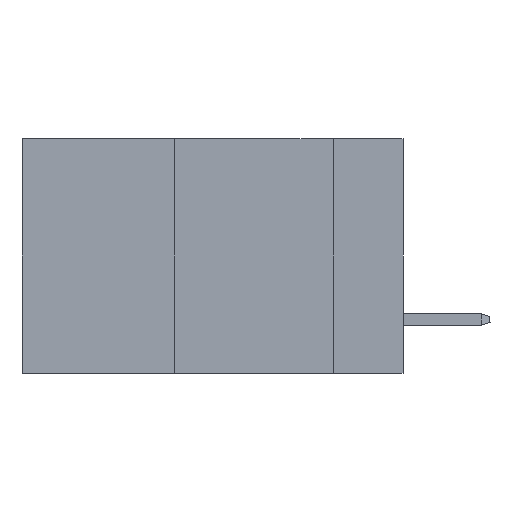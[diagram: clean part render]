
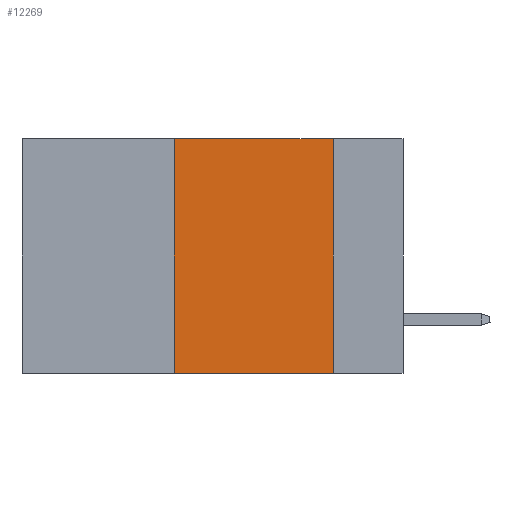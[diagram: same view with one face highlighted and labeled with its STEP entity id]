
A CAD part, left-side view. The second image highlights one B-rep face of the part: STEP entity #12269.
In plain terms, the highlighted planar face has unit normal (-1, 0, 0).
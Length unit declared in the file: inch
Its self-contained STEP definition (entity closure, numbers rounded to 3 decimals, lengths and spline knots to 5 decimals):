
#162 = EDGE_LOOP ( 'NONE', ( #5747, #27386, #3917, #1760 ) ) ;
#396 = CARTESIAN_POINT ( 'NONE',  ( 0., 0.36, 0. ) ) ;
#1760 = ORIENTED_EDGE ( 'NONE', *, *, #8632, .T. ) ;
#2585 = LINE ( 'NONE', #21862, #10414 ) ;
#3626 = DIRECTION ( 'NONE',  ( 1., 0., 0. ) ) ;
#3917 = ORIENTED_EDGE ( 'NONE', *, *, #31104, .F. ) ;
#4366 = CARTESIAN_POINT ( 'NONE',  ( 0., 0.6, 0. ) ) ;
#5747 = ORIENTED_EDGE ( 'NONE', *, *, #14484, .F. ) ;
#6063 = CARTESIAN_POINT ( 'NONE',  ( 0., 0.36, 0. ) ) ;
#7553 = CARTESIAN_POINT ( 'NONE',  ( 0., 0.11, 0. ) ) ;
#8632 = EDGE_CURVE ( 'NONE', #17035, #16111, #31077, .T. ) ;
#9262 = DIRECTION ( 'NONE',  ( 0., 0., 1. ) ) ;
#10414 = VECTOR ( 'NONE', #18802, 39.37008 ) ;
#11462 = VECTOR ( 'NONE', #28971, 39.37008 ) ;
#12269 = ADVANCED_FACE ( 'NONE', ( #25772 ), #20019, .F. ) ;
#13290 = CARTESIAN_POINT ( 'NONE',  ( 0., 0.36, -0.37 ) ) ;
#13818 = VERTEX_POINT ( 'NONE', #396 ) ;
#14210 = VECTOR ( 'NONE', #28398, 39.37008 ) ;
#14484 = EDGE_CURVE ( 'NONE', #14734, #16111, #23923, .T. ) ;
#14734 = VERTEX_POINT ( 'NONE', #22457 ) ;
#14768 = DIRECTION ( 'NONE',  ( 0., 0., -1. ) ) ;
#16111 = VERTEX_POINT ( 'NONE', #18319 ) ;
#17035 = VERTEX_POINT ( 'NONE', #13290 ) ;
#17423 = CARTESIAN_POINT ( 'NONE',  ( 0., 0.6, -0.37 ) ) ;
#18319 = CARTESIAN_POINT ( 'NONE',  ( 0., 0.11, -0.37 ) ) ;
#18802 = DIRECTION ( 'NONE',  ( 0., -1., 0. ) ) ;
#20019 = PLANE ( 'NONE',  #31190 ) ;
#21862 = CARTESIAN_POINT ( 'NONE',  ( 0., 0.6, 0. ) ) ;
#22457 = CARTESIAN_POINT ( 'NONE',  ( 0., 0.11, 0. ) ) ;
#23339 = EDGE_CURVE ( 'NONE', #13818, #14734, #2585, .T. ) ;
#23923 = LINE ( 'NONE', #7553, #11462 ) ;
#25772 = FACE_OUTER_BOUND ( 'NONE', #162, .T. ) ;
#27386 = ORIENTED_EDGE ( 'NONE', *, *, #23339, .F. ) ;
#28398 = DIRECTION ( 'NONE',  ( 0., -1., 0. ) ) ;
#28971 = DIRECTION ( 'NONE',  ( 0., 0., -1. ) ) ;
#31077 = LINE ( 'NONE', #17423, #14210 ) ;
#31104 = EDGE_CURVE ( 'NONE', #17035, #13818, #33907, .T. ) ;
#31146 = VECTOR ( 'NONE', #9262, 39.37008 ) ;
#31190 = AXIS2_PLACEMENT_3D ( 'NONE', #4366, #3626, #14768 ) ;
#33907 = LINE ( 'NONE', #6063, #31146 ) ;
